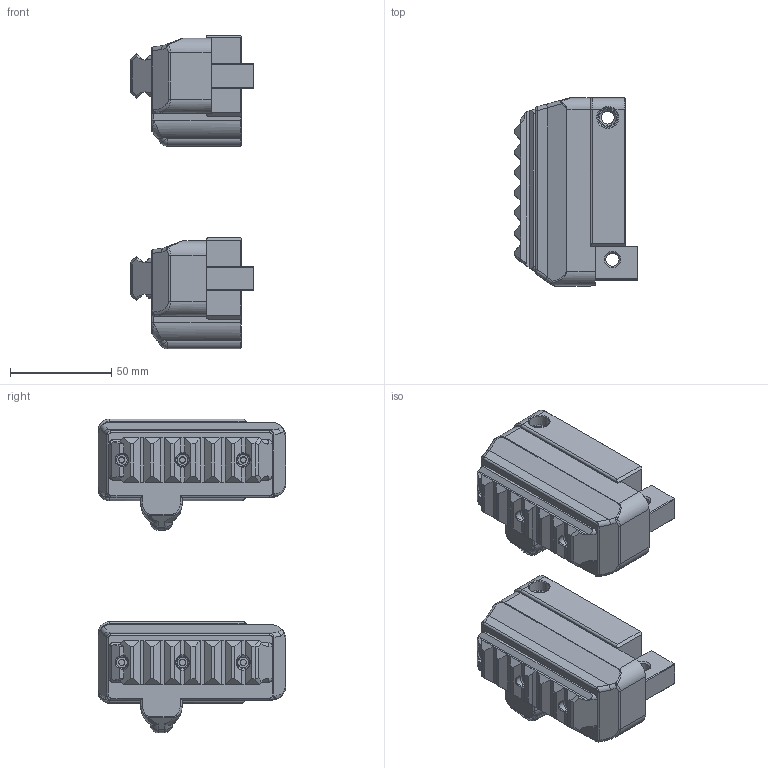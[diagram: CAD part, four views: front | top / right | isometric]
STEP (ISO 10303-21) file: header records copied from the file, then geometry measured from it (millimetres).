
FILE_DESCRIPTION(/* description */ (''),/* implementation_level */ '2;1');
FILE_NAME(/* name */ 'short endcaps.stp',/* time_stamp */ '2021-05-07T02:21:34+02:00',/* author */ (''),/* organization */ (''),/* preprocessor_version */ 'ST-DEVELOPER v15.2',/* originating_system */ 'Autodesk Translator Framework v2.0.0.5431',/* authorisation */ '');
FILE_SCHEMA (('AUTOMOTIVE_DESIGN { 1 0 10303 214 3 1 1 }'));
Length unit declared in the file: centimetre
Products named in the file (1): MOD9 V2 and V3 Short Endcaps
Bounding box: 60.62 x 92.64 x 154.82 mm (x, y, z)
Volume: 267520.3 mm3; surface area: 61669 mm2
Topology: 4 solids, 4 shells, 571 faces, 1445 edges, 891 vertices
Faces by surface type: plane 295, cylinder 124, bspline 79, cone 41, torus 28, sphere 4
Full cylindrical faces by diameter (mm): 2.8 x3, 2.9 x3, 3.1 x6, 4 x1, 6.5 x10, 10 x4, 13 x2, 23.4 x1, 27.4 x1, 27.736 x1
Entity records: 20428 total; most frequent: CARTESIAN_POINT 7398, ORIENTED_EDGE 2714, DIRECTION 2535, EDGE_CURVE 1357, VERTEX_POINT 868, AXIS2_PLACEMENT_3D 855, LINE 825, VECTOR 825
